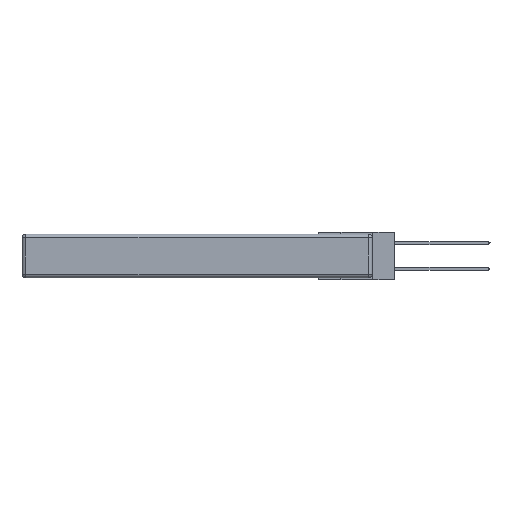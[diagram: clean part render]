
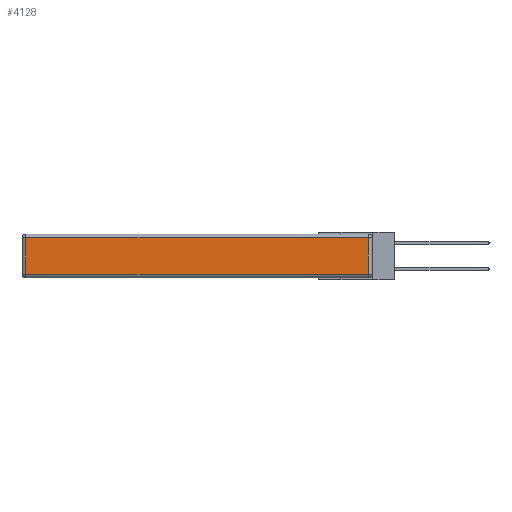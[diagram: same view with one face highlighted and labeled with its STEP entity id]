
A CAD part, left-side view. The second image highlights one B-rep face of the part: STEP entity #4128.
In plain terms, the highlighted planar face has unit normal (-1, 0, 0).
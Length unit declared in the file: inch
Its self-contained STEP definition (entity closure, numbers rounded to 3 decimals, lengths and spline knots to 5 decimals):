
#131 = ORIENTED_EDGE ( 'NONE', *, *, #8153, .T. ) ;
#666 = ORIENTED_EDGE ( 'NONE', *, *, #3763, .T. ) ;
#1300 = ORIENTED_EDGE ( 'NONE', *, *, #7707, .T. ) ;
#1390 = LINE ( 'NONE', #9303, #8256 ) ;
#3763 = EDGE_CURVE ( 'NONE', #7802, #12350, #1390, .T. ) ;
#3903 = DIRECTION ( 'NONE',  ( 0., 0., 1. ) ) ;
#4010 = AXIS2_PLACEMENT_3D ( 'NONE', #10690, #11467, #12469 ) ;
#4128 = ADVANCED_FACE ( 'NONE', ( #7915 ), #9688, .T. ) ;
#5525 = DIRECTION ( 'NONE',  ( 0., 1., 0. ) ) ;
#6110 = VECTOR ( 'NONE', #3903, 39.37008 ) ;
#6141 = CARTESIAN_POINT ( 'NONE',  ( 0., 2.72, -0.313 ) ) ;
#6238 = DIRECTION ( 'NONE',  ( 0., 0., -1. ) ) ;
#6734 = LINE ( 'NONE', #11454, #12504 ) ;
#7254 = EDGE_LOOP ( 'NONE', ( #131, #9639, #1300, #666 ) ) ;
#7323 = CARTESIAN_POINT ( 'NONE',  ( 0., 0.03, -0.313 ) ) ;
#7707 = EDGE_CURVE ( 'NONE', #12239, #7802, #6734, .T. ) ;
#7802 = VERTEX_POINT ( 'NONE', #10098 ) ;
#7915 = FACE_OUTER_BOUND ( 'NONE', #7254, .T. ) ;
#8036 = DIRECTION ( 'NONE',  ( 0., -1., 0. ) ) ;
#8153 = EDGE_CURVE ( 'NONE', #12350, #10776, #10785, .T. ) ;
#8256 = VECTOR ( 'NONE', #6238, 39.37008 ) ;
#8591 = EDGE_CURVE ( 'NONE', #10776, #12239, #8737, .T. ) ;
#8737 = LINE ( 'NONE', #12138, #6110 ) ;
#9303 = CARTESIAN_POINT ( 'NONE',  ( 0., 2.72, -0.343 ) ) ;
#9639 = ORIENTED_EDGE ( 'NONE', *, *, #8591, .T. ) ;
#9688 = PLANE ( 'NONE',  #4010 ) ;
#10098 = CARTESIAN_POINT ( 'NONE',  ( 0., 2.72, -0.03 ) ) ;
#10690 = CARTESIAN_POINT ( 'NONE',  ( 0., 0., -0.343 ) ) ;
#10776 = VERTEX_POINT ( 'NONE', #7323 ) ;
#10785 = LINE ( 'NONE', #11120, #12343 ) ;
#11120 = CARTESIAN_POINT ( 'NONE',  ( 0., 0., -0.313 ) ) ;
#11454 = CARTESIAN_POINT ( 'NONE',  ( 0., 2.75, -0.03 ) ) ;
#11467 = DIRECTION ( 'NONE',  ( -1., 0., 0. ) ) ;
#12138 = CARTESIAN_POINT ( 'NONE',  ( 0., 0.03, -0.343 ) ) ;
#12239 = VERTEX_POINT ( 'NONE', #12854 ) ;
#12343 = VECTOR ( 'NONE', #8036, 39.37008 ) ;
#12350 = VERTEX_POINT ( 'NONE', #6141 ) ;
#12469 = DIRECTION ( 'NONE',  ( 0., 0., 1. ) ) ;
#12504 = VECTOR ( 'NONE', #5525, 39.37008 ) ;
#12854 = CARTESIAN_POINT ( 'NONE',  ( 0., 0.03, -0.03 ) ) ;
